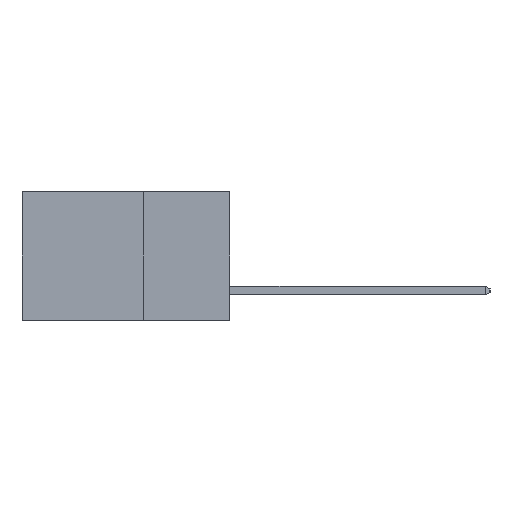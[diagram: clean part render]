
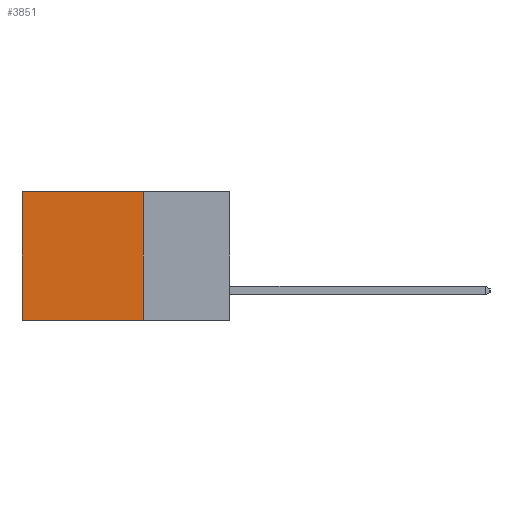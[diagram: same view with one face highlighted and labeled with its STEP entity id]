
A CAD part, left-side view. The second image highlights one B-rep face of the part: STEP entity #3851.
In plain terms, the highlighted planar face has unit normal (-1, 0, 0).
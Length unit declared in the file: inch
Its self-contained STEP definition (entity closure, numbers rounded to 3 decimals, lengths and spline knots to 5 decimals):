
#3062 = CARTESIAN_POINT ( 'NONE',  ( 0.298, 0.6, 0. ) ) ;
#3148 = AXIS2_PLACEMENT_3D ( 'NONE', #11462, #23804, #23504 ) ;
#3577 = ORIENTED_EDGE ( 'NONE', *, *, #20156, .F. ) ;
#3851 = ADVANCED_FACE ( 'NONE', ( #4571 ), #12430, .F. ) ;
#4040 = VERTEX_POINT ( 'NONE', #6425 ) ;
#4159 = VECTOR ( 'NONE', #18010, 39.37008 ) ;
#4571 = FACE_OUTER_BOUND ( 'NONE', #6775, .T. ) ;
#6425 = CARTESIAN_POINT ( 'NONE',  ( 0.298, 0.25, -0.37 ) ) ;
#6775 = EDGE_LOOP ( 'NONE', ( #19662, #14449, #3577, #27035 ) ) ;
#6992 = VERTEX_POINT ( 'NONE', #3062 ) ;
#7182 = EDGE_CURVE ( 'NONE', #6992, #8666, #27534, .T. ) ;
#8665 = LINE ( 'NONE', #13990, #25117 ) ;
#8666 = VERTEX_POINT ( 'NONE', #19805 ) ;
#10013 = LINE ( 'NONE', #11500, #4159 ) ;
#11462 = CARTESIAN_POINT ( 'NONE',  ( 0.298, 0.25, 0. ) ) ;
#11500 = CARTESIAN_POINT ( 'NONE',  ( 0.298, 0.25, 0. ) ) ;
#12075 = CARTESIAN_POINT ( 'NONE',  ( 0.298, 0.25, -0.37 ) ) ;
#12430 = PLANE ( 'NONE',  #3148 ) ;
#12458 = CARTESIAN_POINT ( 'NONE',  ( 0.298, 0.25, 0. ) ) ;
#13990 = CARTESIAN_POINT ( 'NONE',  ( 0.298, 0.25, 0. ) ) ;
#14449 = ORIENTED_EDGE ( 'NONE', *, *, #20257, .F. ) ;
#16146 = DIRECTION ( 'NONE',  ( 0., 0., -1. ) ) ;
#16866 = VECTOR ( 'NONE', #20669, 39.37008 ) ;
#17526 = LINE ( 'NONE', #12075, #16866 ) ;
#18010 = DIRECTION ( 'NONE',  ( 0., 1., 0. ) ) ;
#19662 = ORIENTED_EDGE ( 'NONE', *, *, #7182, .T. ) ;
#19805 = CARTESIAN_POINT ( 'NONE',  ( 0.298, 0.6, -0.37 ) ) ;
#20156 = EDGE_CURVE ( 'NONE', #23856, #4040, #8665, .T. ) ;
#20257 = EDGE_CURVE ( 'NONE', #4040, #8666, #17526, .T. ) ;
#20669 = DIRECTION ( 'NONE',  ( 0., 1., 0. ) ) ;
#21917 = VECTOR ( 'NONE', #23308, 39.37008 ) ;
#23308 = DIRECTION ( 'NONE',  ( 0., 0., -1. ) ) ;
#23504 = DIRECTION ( 'NONE',  ( 0., 0., -1. ) ) ;
#23804 = DIRECTION ( 'NONE',  ( 1., 0., 0. ) ) ;
#23856 = VERTEX_POINT ( 'NONE', #12458 ) ;
#25117 = VECTOR ( 'NONE', #16146, 39.37008 ) ;
#25581 = CARTESIAN_POINT ( 'NONE',  ( 0.298, 0.6, 0. ) ) ;
#26084 = EDGE_CURVE ( 'NONE', #23856, #6992, #10013, .T. ) ;
#27035 = ORIENTED_EDGE ( 'NONE', *, *, #26084, .T. ) ;
#27534 = LINE ( 'NONE', #25581, #21917 ) ;
